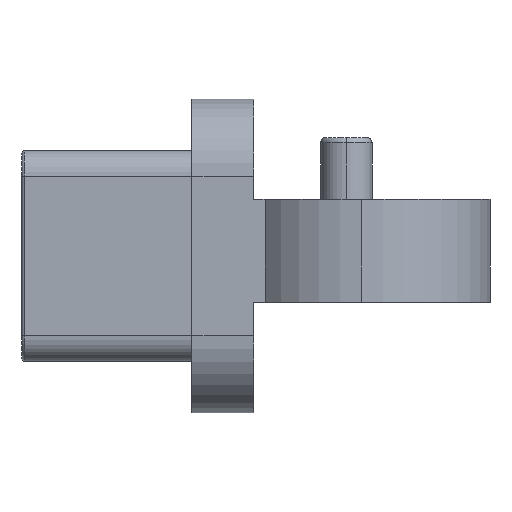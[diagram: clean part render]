
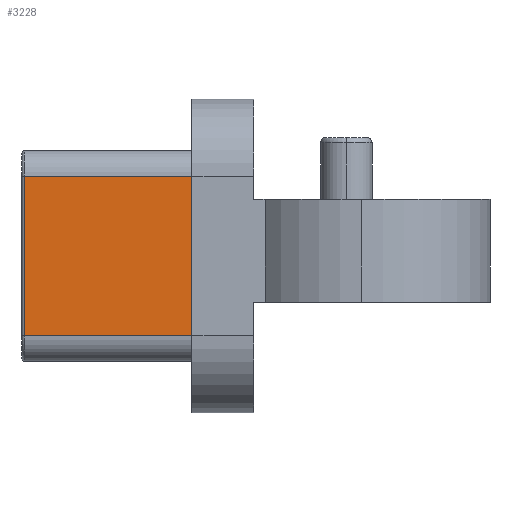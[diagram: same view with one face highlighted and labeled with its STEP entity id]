
A CAD part, left-side view. The second image highlights one B-rep face of the part: STEP entity #3228.
In plain terms, the highlighted planar face has unit normal (-1, 0, 0).
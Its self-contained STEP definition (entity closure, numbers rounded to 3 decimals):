
#902 = LINE ( 'NONE', #4930, #3980 ) ;
#922 = DIRECTION ( 'NONE',  ( 0., -1., 0. ) ) ;
#952 = PLANE ( 'NONE',  #6185 ) ;
#1051 = DIRECTION ( 'NONE',  ( 0., 0., -1. ) ) ;
#1559 = CARTESIAN_POINT ( 'NONE',  ( -9.65, 1.2, 1.55 ) ) ;
#1628 = DIRECTION ( 'NONE',  ( 1., 0., 0. ) ) ;
#1821 = CARTESIAN_POINT ( 'NONE',  ( -9.65, 4.45, 2.05 ) ) ;
#1906 = CARTESIAN_POINT ( 'NONE',  ( -9.65, 1.2, -1.55 ) ) ;
#2301 = EDGE_CURVE ( 'NONE', #6514, #3349, #4110, .T. ) ;
#2424 = LINE ( 'NONE', #5085, #4105 ) ;
#2796 = EDGE_LOOP ( 'NONE', ( #4387, #2971, #2978, #4394 ) ) ;
#2884 = EDGE_CURVE ( 'NONE', #3033, #3255, #5330, .T. ) ;
#2971 = ORIENTED_EDGE ( 'NONE', *, *, #2301, .T. ) ;
#2978 = ORIENTED_EDGE ( 'NONE', *, *, #3111, .T. ) ;
#3033 = VERTEX_POINT ( 'NONE', #1906 ) ;
#3111 = EDGE_CURVE ( 'NONE', #3349, #3033, #2424, .T. ) ;
#3228 = ADVANCED_FACE ( 'NONE', ( #4223 ), #952, .F. ) ;
#3255 = VERTEX_POINT ( 'NONE', #1559 ) ;
#3349 = VERTEX_POINT ( 'NONE', #5938 ) ;
#3647 = EDGE_CURVE ( 'NONE', #3255, #6514, #902, .T. ) ;
#3980 = VECTOR ( 'NONE', #5483, 1000. ) ;
#4105 = VECTOR ( 'NONE', #922, 1000. ) ;
#4110 = LINE ( 'NONE', #1821, #5362 ) ;
#4223 = FACE_OUTER_BOUND ( 'NONE', #2796, .T. ) ;
#4266 = CARTESIAN_POINT ( 'NONE',  ( -9.65, 1.2, 2.05 ) ) ;
#4294 = CARTESIAN_POINT ( 'NONE',  ( -9.65, 4.45, 1.55 ) ) ;
#4387 = ORIENTED_EDGE ( 'NONE', *, *, #3647, .T. ) ;
#4394 = ORIENTED_EDGE ( 'NONE', *, *, #2884, .T. ) ;
#4747 = DIRECTION ( 'NONE',  ( 0., 0., 1. ) ) ;
#4930 = CARTESIAN_POINT ( 'NONE',  ( -9.65, 4.5, 1.55 ) ) ;
#4968 = VECTOR ( 'NONE', #4747, 1000. ) ;
#5085 = CARTESIAN_POINT ( 'NONE',  ( -9.65, 4.5, -1.55 ) ) ;
#5187 = CARTESIAN_POINT ( 'NONE',  ( -9.65, 4.5, 2.05 ) ) ;
#5330 = LINE ( 'NONE', #4266, #4968 ) ;
#5362 = VECTOR ( 'NONE', #6202, 1000. ) ;
#5483 = DIRECTION ( 'NONE',  ( 0., 1., 0. ) ) ;
#5938 = CARTESIAN_POINT ( 'NONE',  ( -9.65, 4.45, -1.55 ) ) ;
#6185 = AXIS2_PLACEMENT_3D ( 'NONE', #5187, #1628, #1051 ) ;
#6202 = DIRECTION ( 'NONE',  ( 0., 0., -1. ) ) ;
#6514 = VERTEX_POINT ( 'NONE', #4294 ) ;
